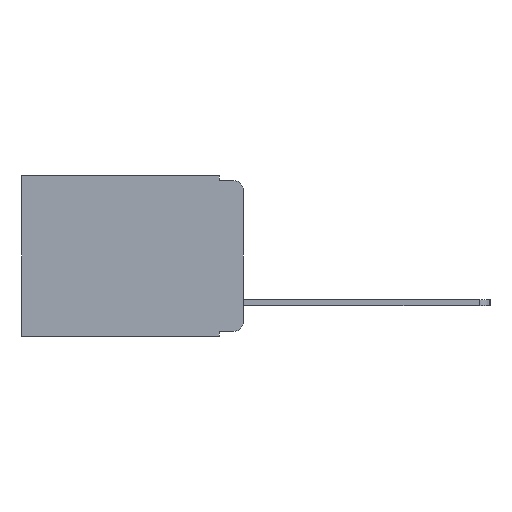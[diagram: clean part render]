
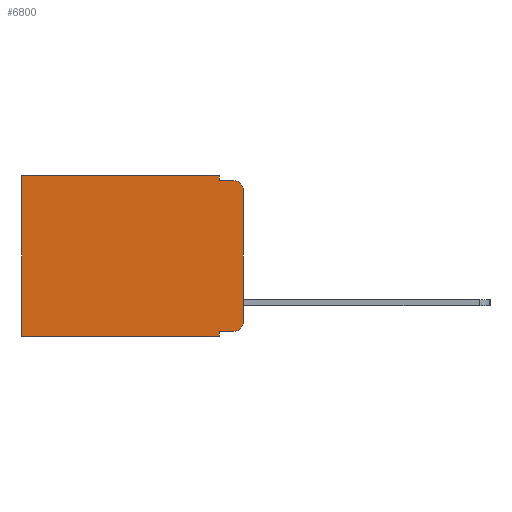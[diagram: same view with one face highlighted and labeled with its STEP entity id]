
A CAD part, left-side view. The second image highlights one B-rep face of the part: STEP entity #6800.
In plain terms, the highlighted planar face has unit normal (-1, 0, 0).
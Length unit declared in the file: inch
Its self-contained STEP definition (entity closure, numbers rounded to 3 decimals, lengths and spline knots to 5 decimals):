
#253 = EDGE_CURVE ( 'NONE', #1115, #9638, #3033, .T. ) ;
#422 = CIRCLE ( 'NONE', #11398, 0.02 ) ;
#711 = ORIENTED_EDGE ( 'NONE', *, *, #10394, .F. ) ;
#961 = CARTESIAN_POINT ( 'NONE',  ( 0.298, 0.051, 0. ) ) ;
#969 = ORIENTED_EDGE ( 'NONE', *, *, #253, .T. ) ;
#985 = CARTESIAN_POINT ( 'NONE',  ( 0.298, 0., 0. ) ) ;
#1028 = VECTOR ( 'NONE', #10371, 39.37008 ) ;
#1115 = VERTEX_POINT ( 'NONE', #11629 ) ;
#1366 = VERTEX_POINT ( 'NONE', #11953 ) ;
#1478 = CARTESIAN_POINT ( 'NONE',  ( 0.298, 0.051, -0.333 ) ) ;
#1946 = EDGE_CURVE ( 'NONE', #1366, #1115, #12946, .T. ) ;
#2323 = DIRECTION ( 'NONE',  ( 0., 0., -1. ) ) ;
#2454 = ORIENTED_EDGE ( 'NONE', *, *, #3827, .F. ) ;
#2854 = ORIENTED_EDGE ( 'NONE', *, *, #12533, .T. ) ;
#3033 = LINE ( 'NONE', #4287, #5814 ) ;
#3193 = FACE_OUTER_BOUND ( 'NONE', #8311, .T. ) ;
#3359 = VECTOR ( 'NONE', #2323, 39.37008 ) ;
#3468 = EDGE_CURVE ( 'NONE', #13182, #9638, #12725, .T. ) ;
#3500 = DIRECTION ( 'NONE',  ( 0., 1., 0. ) ) ;
#3513 = CARTESIAN_POINT ( 'NONE',  ( 0.298, 0., -0.343 ) ) ;
#3791 = CARTESIAN_POINT ( 'NONE',  ( 0.298, 0., 0. ) ) ;
#3827 = EDGE_CURVE ( 'NONE', #7621, #9375, #9744, .T. ) ;
#3932 = DIRECTION ( 'NONE',  ( 0., 1., 0. ) ) ;
#4051 = DIRECTION ( 'NONE',  ( -1., 0., 0. ) ) ;
#4104 = CARTESIAN_POINT ( 'NONE',  ( 0.298, 0.02, -0.03 ) ) ;
#4142 = LINE ( 'NONE', #961, #3359 ) ;
#4287 = CARTESIAN_POINT ( 'NONE',  ( 0.298, 0.473, 0. ) ) ;
#4291 = CARTESIAN_POINT ( 'NONE',  ( 0.298, 0.051, -0.01 ) ) ;
#4602 = ORIENTED_EDGE ( 'NONE', *, *, #10161, .F. ) ;
#5142 = CARTESIAN_POINT ( 'NONE',  ( 0.298, 0.473, -0.343 ) ) ;
#5254 = DIRECTION ( 'NONE',  ( 0., 0., -1. ) ) ;
#5654 = ORIENTED_EDGE ( 'NONE', *, *, #8707, .F. ) ;
#5689 = ORIENTED_EDGE ( 'NONE', *, *, #8969, .T. ) ;
#5767 = VERTEX_POINT ( 'NONE', #11843 ) ;
#5814 = VECTOR ( 'NONE', #7281, 39.37008 ) ;
#5997 = VECTOR ( 'NONE', #11994, 39.37008 ) ;
#6549 = DIRECTION ( 'NONE',  ( 0., 0., -1. ) ) ;
#6800 = ADVANCED_FACE ( 'NONE', ( #3193 ), #13599, .F. ) ;
#6919 = CARTESIAN_POINT ( 'NONE',  ( 0.298, 0., -0.313 ) ) ;
#7281 = DIRECTION ( 'NONE',  ( 0., 0., -1. ) ) ;
#7333 = LINE ( 'NONE', #13887, #12710 ) ;
#7439 = DIRECTION ( 'NONE',  ( 0., -1., 0. ) ) ;
#7621 = VERTEX_POINT ( 'NONE', #4291 ) ;
#8311 = EDGE_LOOP ( 'NONE', ( #4602, #10022, #2454, #5654, #13731, #969, #12500, #711, #2854, #5689 ) ) ;
#8707 = EDGE_CURVE ( 'NONE', #1366, #7621, #4142, .T. ) ;
#8969 = EDGE_CURVE ( 'NONE', #5767, #11420, #422, .T. ) ;
#9375 = VERTEX_POINT ( 'NONE', #12290 ) ;
#9638 = VERTEX_POINT ( 'NONE', #5142 ) ;
#9744 = LINE ( 'NONE', #10112, #10553 ) ;
#9798 = VECTOR ( 'NONE', #3932, 39.37008 ) ;
#10022 = ORIENTED_EDGE ( 'NONE', *, *, #11175, .T. ) ;
#10112 = CARTESIAN_POINT ( 'NONE',  ( 0.298, 0.051, -0.01 ) ) ;
#10161 = EDGE_CURVE ( 'NONE', #11404, #11420, #13242, .T. ) ;
#10371 = DIRECTION ( 'NONE',  ( 0., 0., -1. ) ) ;
#10394 = EDGE_CURVE ( 'NONE', #11185, #13182, #7333, .T. ) ;
#10553 = VECTOR ( 'NONE', #7439, 39.37008 ) ;
#10714 = CARTESIAN_POINT ( 'NONE',  ( 0.298, 0.02, -0.313 ) ) ;
#10912 = CARTESIAN_POINT ( 'NONE',  ( 0.298, 0.051, -0.333 ) ) ;
#11175 = EDGE_CURVE ( 'NONE', #11404, #9375, #11864, .T. ) ;
#11185 = VERTEX_POINT ( 'NONE', #1478 ) ;
#11370 = DIRECTION ( 'NONE',  ( 1., 0., 0. ) ) ;
#11398 = AXIS2_PLACEMENT_3D ( 'NONE', #10714, #4051, #11791 ) ;
#11404 = VERTEX_POINT ( 'NONE', #14468 ) ;
#11420 = VERTEX_POINT ( 'NONE', #6919 ) ;
#11629 = CARTESIAN_POINT ( 'NONE',  ( 0.298, 0.473, 0. ) ) ;
#11720 = DIRECTION ( 'NONE',  ( 0., 0., -1. ) ) ;
#11791 = DIRECTION ( 'NONE',  ( 0., 0., -1. ) ) ;
#11843 = CARTESIAN_POINT ( 'NONE',  ( 0.298, 0.02, -0.333 ) ) ;
#11846 = DIRECTION ( 'NONE',  ( -1., 0., 0. ) ) ;
#11864 = CIRCLE ( 'NONE', #14952, 0.02 ) ;
#11953 = CARTESIAN_POINT ( 'NONE',  ( 0.298, 0.051, 0. ) ) ;
#11994 = DIRECTION ( 'NONE',  ( 0., -1., 0. ) ) ;
#12290 = CARTESIAN_POINT ( 'NONE',  ( 0.298, 0.02, -0.01 ) ) ;
#12500 = ORIENTED_EDGE ( 'NONE', *, *, #3468, .F. ) ;
#12533 = EDGE_CURVE ( 'NONE', #11185, #5767, #14707, .T. ) ;
#12710 = VECTOR ( 'NONE', #11720, 39.37008 ) ;
#12725 = LINE ( 'NONE', #3513, #13071 ) ;
#12946 = LINE ( 'NONE', #3791, #9798 ) ;
#13071 = VECTOR ( 'NONE', #3500, 39.37008 ) ;
#13182 = VERTEX_POINT ( 'NONE', #14085 ) ;
#13242 = LINE ( 'NONE', #985, #1028 ) ;
#13599 = PLANE ( 'NONE',  #13955 ) ;
#13731 = ORIENTED_EDGE ( 'NONE', *, *, #1946, .T. ) ;
#13887 = CARTESIAN_POINT ( 'NONE',  ( 0.298, 0.051, 0. ) ) ;
#13955 = AXIS2_PLACEMENT_3D ( 'NONE', #14378, #11370, #6549 ) ;
#14085 = CARTESIAN_POINT ( 'NONE',  ( 0.298, 0.051, -0.343 ) ) ;
#14378 = CARTESIAN_POINT ( 'NONE',  ( 0.298, 0., 0. ) ) ;
#14468 = CARTESIAN_POINT ( 'NONE',  ( 0.298, 0., -0.03 ) ) ;
#14707 = LINE ( 'NONE', #10912, #5997 ) ;
#14952 = AXIS2_PLACEMENT_3D ( 'NONE', #4104, #11846, #5254 ) ;
